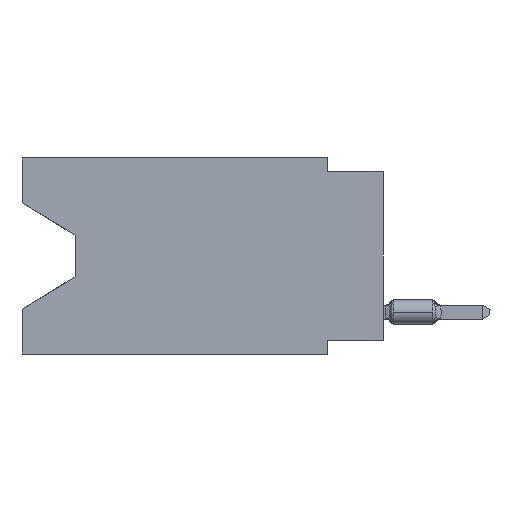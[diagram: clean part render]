
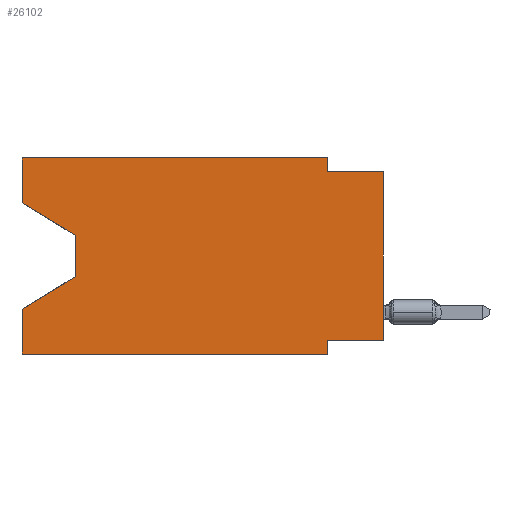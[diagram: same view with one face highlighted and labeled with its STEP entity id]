
A CAD part, left-side view. The second image highlights one B-rep face of the part: STEP entity #26102.
In plain terms, the highlighted planar face has unit normal (-1, 0, 0).
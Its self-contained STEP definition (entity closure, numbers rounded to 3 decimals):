
#218 = CARTESIAN_POINT ( 'NONE',  ( 0., 13.97, -5.385 ) ) ;
#671 = VERTEX_POINT ( 'NONE', #32810 ) ;
#689 = EDGE_CURVE ( 'NONE', #12167, #29875, #30425, .T. ) ;
#717 = LINE ( 'NONE', #11076, #29397 ) ;
#840 = ORIENTED_EDGE ( 'NONE', *, *, #1142, .T. ) ;
#1039 = AXIS2_PLACEMENT_3D ( 'NONE', #31550, #18642, #23393 ) ;
#1142 = EDGE_CURVE ( 'NONE', #32628, #7154, #18789, .T. ) ;
#2059 = VERTEX_POINT ( 'NONE', #17634 ) ;
#2265 = DIRECTION ( 'NONE',  ( 0., -1., 0. ) ) ;
#2515 = LINE ( 'NONE', #8264, #4282 ) ;
#3330 = DIRECTION ( 'NONE',  ( 0., 0., 1. ) ) ;
#3755 = DIRECTION ( 'NONE',  ( 0., -1., 0. ) ) ;
#3925 = EDGE_LOOP ( 'NONE', ( #8540, #29849, #16249, #8325, #26063, #6849, #32269, #840, #7923, #19861, #24927, #11291 ) ) ;
#4139 = DIRECTION ( 'NONE',  ( 0., -0.855, -0.519 ) ) ;
#4282 = VECTOR ( 'NONE', #33423, 1000. ) ;
#4524 = CARTESIAN_POINT ( 'NONE',  ( 0., 0., -0.635 ) ) ;
#5558 = LINE ( 'NONE', #15940, #27853 ) ;
#5652 = VERTEX_POINT ( 'NONE', #11479 ) ;
#5966 = DIRECTION ( 'NONE',  ( 0., 0., -1. ) ) ;
#6510 = LINE ( 'NONE', #19434, #17616 ) ;
#6849 = ORIENTED_EDGE ( 'NONE', *, *, #689, .F. ) ;
#6995 = EDGE_CURVE ( 'NONE', #12735, #2059, #5558, .T. ) ;
#7154 = VERTEX_POINT ( 'NONE', #4524 ) ;
#7476 = VECTOR ( 'NONE', #25668, 1000. ) ;
#7923 = ORIENTED_EDGE ( 'NONE', *, *, #29641, .F. ) ;
#8011 = LINE ( 'NONE', #218, #18523 ) ;
#8039 = VECTOR ( 'NONE', #5966, 1000. ) ;
#8264 = CARTESIAN_POINT ( 'NONE',  ( 0., 2.54, 0. ) ) ;
#8325 = ORIENTED_EDGE ( 'NONE', *, *, #25430, .F. ) ;
#8540 = ORIENTED_EDGE ( 'NONE', *, *, #10075, .T. ) ;
#8715 = VECTOR ( 'NONE', #2265, 1000. ) ;
#9000 = CARTESIAN_POINT ( 'NONE',  ( 0., 16.383, -2.038 ) ) ;
#9468 = LINE ( 'NONE', #14228, #14383 ) ;
#9586 = CARTESIAN_POINT ( 'NONE',  ( 0., 2.54, -8.255 ) ) ;
#10075 = EDGE_CURVE ( 'NONE', #18469, #671, #6510, .T. ) ;
#10703 = CARTESIAN_POINT ( 'NONE',  ( 0., 13.97, -5.385 ) ) ;
#10976 = VERTEX_POINT ( 'NONE', #10703 ) ;
#11076 = CARTESIAN_POINT ( 'NONE',  ( 0., 16.383, -8.89 ) ) ;
#11195 = CARTESIAN_POINT ( 'NONE',  ( 0., 16.383, -8.89 ) ) ;
#11291 = ORIENTED_EDGE ( 'NONE', *, *, #18791, .F. ) ;
#11479 = CARTESIAN_POINT ( 'NONE',  ( 0., 16.383, -6.852 ) ) ;
#11678 = CARTESIAN_POINT ( 'NONE',  ( 0., 2.54, -8.89 ) ) ;
#11948 = VECTOR ( 'NONE', #19925, 1000. ) ;
#12110 = CARTESIAN_POINT ( 'NONE',  ( 0., 0., -8.255 ) ) ;
#12167 = VERTEX_POINT ( 'NONE', #9586 ) ;
#12225 = LINE ( 'NONE', #25972, #19120 ) ;
#12735 = VERTEX_POINT ( 'NONE', #31577 ) ;
#14228 = CARTESIAN_POINT ( 'NONE',  ( 0., 16.383, 0. ) ) ;
#14383 = VECTOR ( 'NONE', #32071, 1000. ) ;
#14936 = VERTEX_POINT ( 'NONE', #28766 ) ;
#15129 = CARTESIAN_POINT ( 'NONE',  ( 0., 2.54, -8.89 ) ) ;
#15940 = CARTESIAN_POINT ( 'NONE',  ( 0., 16.383, 0. ) ) ;
#16249 = ORIENTED_EDGE ( 'NONE', *, *, #21104, .T. ) ;
#17545 = LINE ( 'NONE', #12110, #11948 ) ;
#17616 = VECTOR ( 'NONE', #4139, 1000. ) ;
#17634 = CARTESIAN_POINT ( 'NONE',  ( 0., 2.54, 0. ) ) ;
#18469 = VERTEX_POINT ( 'NONE', #9000 ) ;
#18523 = VECTOR ( 'NONE', #26209, 1000. ) ;
#18642 = DIRECTION ( 'NONE',  ( 1., 0., 0. ) ) ;
#18789 = LINE ( 'NONE', #32215, #31395 ) ;
#18791 = EDGE_CURVE ( 'NONE', #18469, #12735, #9468, .T. ) ;
#19120 = VECTOR ( 'NONE', #32947, 1000. ) ;
#19434 = CARTESIAN_POINT ( 'NONE',  ( 0., 16.383, -2.038 ) ) ;
#19716 = EDGE_CURVE ( 'NONE', #32628, #12167, #17545, .T. ) ;
#19861 = ORIENTED_EDGE ( 'NONE', *, *, #26131, .F. ) ;
#19925 = DIRECTION ( 'NONE',  ( 0., 1., 0. ) ) ;
#20519 = FACE_OUTER_BOUND ( 'NONE', #3925, .T. ) ;
#21104 = EDGE_CURVE ( 'NONE', #10976, #5652, #8011, .T. ) ;
#21232 = EDGE_CURVE ( 'NONE', #28683, #29875, #717, .T. ) ;
#21445 = LINE ( 'NONE', #31808, #8039 ) ;
#23393 = DIRECTION ( 'NONE',  ( 0., 0., -1. ) ) ;
#24927 = ORIENTED_EDGE ( 'NONE', *, *, #6995, .F. ) ;
#25430 = EDGE_CURVE ( 'NONE', #28683, #5652, #12225, .T. ) ;
#25668 = DIRECTION ( 'NONE',  ( 0., 0., -1. ) ) ;
#25972 = CARTESIAN_POINT ( 'NONE',  ( 0., 16.383, 0. ) ) ;
#25986 = CARTESIAN_POINT ( 'NONE',  ( 0., 0., -8.255 ) ) ;
#26063 = ORIENTED_EDGE ( 'NONE', *, *, #21232, .T. ) ;
#26102 = ADVANCED_FACE ( 'NONE', ( #20519 ), #28833, .F. ) ;
#26131 = EDGE_CURVE ( 'NONE', #2059, #14936, #2515, .T. ) ;
#26209 = DIRECTION ( 'NONE',  ( 0., 0.855, -0.519 ) ) ;
#26308 = DIRECTION ( 'NONE',  ( 0., -1., 0. ) ) ;
#27172 = EDGE_CURVE ( 'NONE', #671, #10976, #21445, .T. ) ;
#27853 = VECTOR ( 'NONE', #26308, 1000. ) ;
#28435 = LINE ( 'NONE', #33500, #8715 ) ;
#28683 = VERTEX_POINT ( 'NONE', #11195 ) ;
#28766 = CARTESIAN_POINT ( 'NONE',  ( 0., 2.54, -0.635 ) ) ;
#28833 = PLANE ( 'NONE',  #1039 ) ;
#29397 = VECTOR ( 'NONE', #3755, 1000. ) ;
#29641 = EDGE_CURVE ( 'NONE', #14936, #7154, #28435, .T. ) ;
#29849 = ORIENTED_EDGE ( 'NONE', *, *, #27172, .T. ) ;
#29875 = VERTEX_POINT ( 'NONE', #11678 ) ;
#30425 = LINE ( 'NONE', #15129, #7476 ) ;
#31395 = VECTOR ( 'NONE', #3330, 1000. ) ;
#31550 = CARTESIAN_POINT ( 'NONE',  ( 0., 16.383, 0. ) ) ;
#31577 = CARTESIAN_POINT ( 'NONE',  ( 0., 16.383, 0. ) ) ;
#31808 = CARTESIAN_POINT ( 'NONE',  ( 0., 13.97, -3.505 ) ) ;
#32071 = DIRECTION ( 'NONE',  ( 0., 0., 1. ) ) ;
#32215 = CARTESIAN_POINT ( 'NONE',  ( 0., 0., 0. ) ) ;
#32269 = ORIENTED_EDGE ( 'NONE', *, *, #19716, .F. ) ;
#32628 = VERTEX_POINT ( 'NONE', #25986 ) ;
#32810 = CARTESIAN_POINT ( 'NONE',  ( 0., 13.97, -3.505 ) ) ;
#32947 = DIRECTION ( 'NONE',  ( 0., 0., 1. ) ) ;
#33423 = DIRECTION ( 'NONE',  ( 0., 0., -1. ) ) ;
#33500 = CARTESIAN_POINT ( 'NONE',  ( 0., 0., -0.635 ) ) ;
